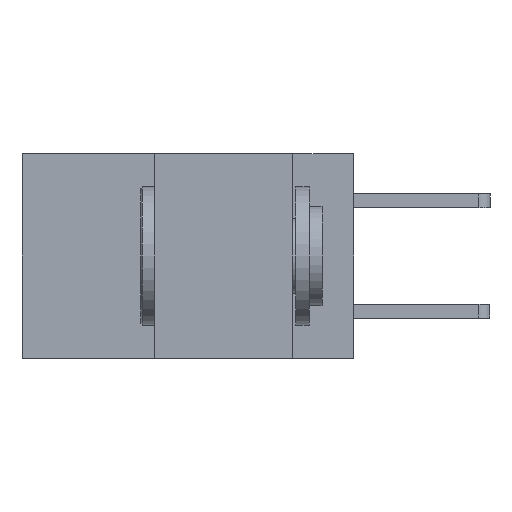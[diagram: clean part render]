
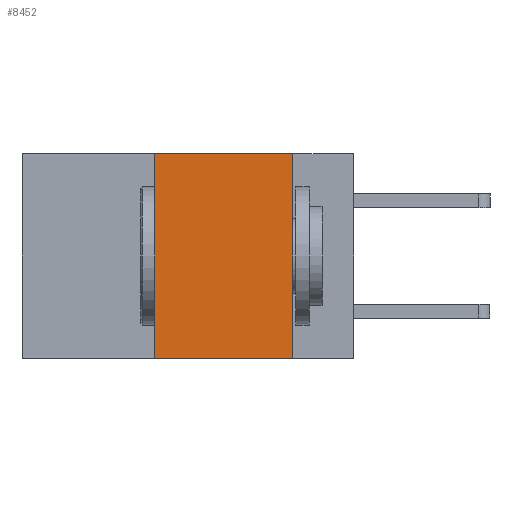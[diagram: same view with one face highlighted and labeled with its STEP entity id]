
A CAD part, left-side view. The second image highlights one B-rep face of the part: STEP entity #8452.
In plain terms, the highlighted planar face has unit normal (-1, 0, 0).
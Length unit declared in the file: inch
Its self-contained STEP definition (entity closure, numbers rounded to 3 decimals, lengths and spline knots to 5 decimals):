
#132 = CARTESIAN_POINT ( 'NONE',  ( 0., 0.6, -0.37 ) ) ;
#146 = DIRECTION ( 'NONE',  ( 1., 0., 0. ) ) ;
#197 = LINE ( 'NONE', #132, #6311 ) ;
#261 = CARTESIAN_POINT ( 'NONE',  ( 0., 0.6, 0. ) ) ;
#379 = VECTOR ( 'NONE', #3370, 39.37008 ) ;
#424 = VECTOR ( 'NONE', #4037, 39.37008 ) ;
#853 = CARTESIAN_POINT ( 'NONE',  ( 0., 0.11, 0. ) ) ;
#910 = LINE ( 'NONE', #853, #2222 ) ;
#1457 = ORIENTED_EDGE ( 'NONE', *, *, #11928, .F. ) ;
#1761 = EDGE_CURVE ( 'NONE', #6375, #5136, #910, .T. ) ;
#2222 = VECTOR ( 'NONE', #2700, 39.37008 ) ;
#2253 = LINE ( 'NONE', #6163, #379 ) ;
#2433 = CARTESIAN_POINT ( 'NONE',  ( 0., 0.11, -0.37 ) ) ;
#2700 = DIRECTION ( 'NONE',  ( 0., 0., -1. ) ) ;
#2738 = VERTEX_POINT ( 'NONE', #10345 ) ;
#2922 = PLANE ( 'NONE',  #10049 ) ;
#3370 = DIRECTION ( 'NONE',  ( 0., 0., 1. ) ) ;
#3454 = ORIENTED_EDGE ( 'NONE', *, *, #8835, .T. ) ;
#4037 = DIRECTION ( 'NONE',  ( 0., -1., 0. ) ) ;
#4049 = CARTESIAN_POINT ( 'NONE',  ( 0., 0.36, 0. ) ) ;
#4110 = CARTESIAN_POINT ( 'NONE',  ( 0., 0.6, 0. ) ) ;
#4355 = ORIENTED_EDGE ( 'NONE', *, *, #1761, .F. ) ;
#4705 = ORIENTED_EDGE ( 'NONE', *, *, #9701, .F. ) ;
#4968 = DIRECTION ( 'NONE',  ( 0., -1., 0. ) ) ;
#5136 = VERTEX_POINT ( 'NONE', #2433 ) ;
#5899 = FACE_OUTER_BOUND ( 'NONE', #6120, .T. ) ;
#6120 = EDGE_LOOP ( 'NONE', ( #4355, #1457, #4705, #3454 ) ) ;
#6163 = CARTESIAN_POINT ( 'NONE',  ( 0., 0.36, 0. ) ) ;
#6311 = VECTOR ( 'NONE', #4968, 39.37008 ) ;
#6375 = VERTEX_POINT ( 'NONE', #8974 ) ;
#7888 = DIRECTION ( 'NONE',  ( 0., 0., -1. ) ) ;
#8452 = ADVANCED_FACE ( 'NONE', ( #5899 ), #2922, .F. ) ;
#8835 = EDGE_CURVE ( 'NONE', #2738, #5136, #197, .T. ) ;
#8974 = CARTESIAN_POINT ( 'NONE',  ( 0., 0.11, 0. ) ) ;
#9701 = EDGE_CURVE ( 'NONE', #2738, #10280, #2253, .T. ) ;
#10049 = AXIS2_PLACEMENT_3D ( 'NONE', #4110, #146, #7888 ) ;
#10280 = VERTEX_POINT ( 'NONE', #4049 ) ;
#10345 = CARTESIAN_POINT ( 'NONE',  ( 0., 0.36, -0.37 ) ) ;
#10424 = LINE ( 'NONE', #261, #424 ) ;
#11928 = EDGE_CURVE ( 'NONE', #10280, #6375, #10424, .T. ) ;
